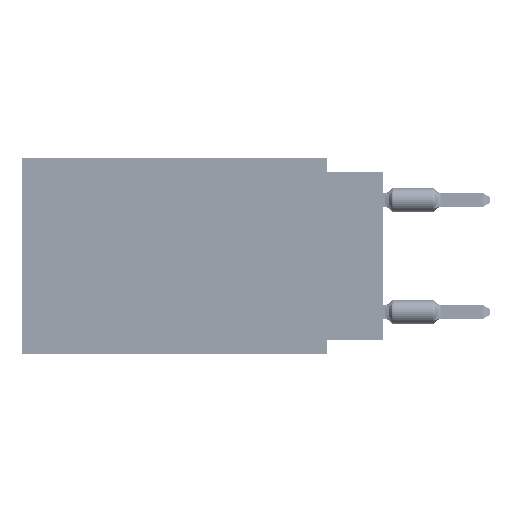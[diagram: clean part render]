
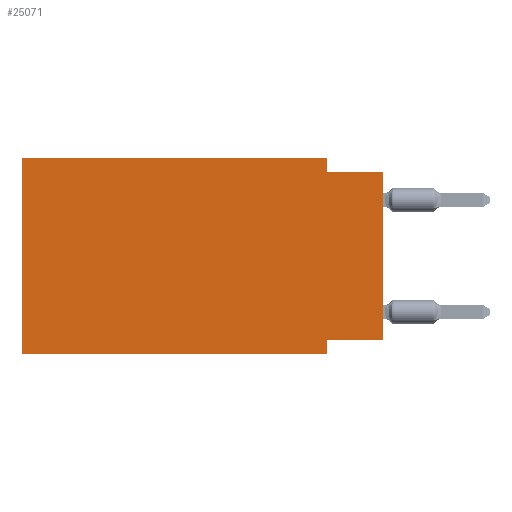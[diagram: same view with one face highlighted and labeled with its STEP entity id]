
A CAD part, left-side view. The second image highlights one B-rep face of the part: STEP entity #25071.
In plain terms, the highlighted planar face has unit normal (-1, 0, 0).
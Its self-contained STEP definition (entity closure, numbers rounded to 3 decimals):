
#673 = CARTESIAN_POINT ( 'NONE',  ( 0., 16.383, -8.89 ) ) ;
#1722 = EDGE_CURVE ( 'NONE', #19170, #26850, #45994, .T. ) ;
#2301 = EDGE_CURVE ( 'NONE', #38487, #80072, #85612, .T. ) ;
#2666 = LINE ( 'NONE', #11563, #86564 ) ;
#3224 = EDGE_CURVE ( 'NONE', #51161, #48623, #49148, .T. ) ;
#7296 = LINE ( 'NONE', #36738, #79432 ) ;
#8355 = DIRECTION ( 'NONE',  ( 0., -1., 0. ) ) ;
#9740 = EDGE_CURVE ( 'NONE', #73928, #40992, #46923, .T. ) ;
#11563 = CARTESIAN_POINT ( 'NONE',  ( 0., 16.383, 0. ) ) ;
#12191 = CARTESIAN_POINT ( 'NONE',  ( 0., 2.54, -8.255 ) ) ;
#13010 = EDGE_CURVE ( 'NONE', #80072, #48623, #7296, .T. ) ;
#15290 = FACE_OUTER_BOUND ( 'NONE', #47581, .T. ) ;
#19170 = VERTEX_POINT ( 'NONE', #38067 ) ;
#19643 = EDGE_CURVE ( 'NONE', #38487, #26850, #84244, .T. ) ;
#20157 = CARTESIAN_POINT ( 'NONE',  ( 0., 0., -0.635 ) ) ;
#23445 = VECTOR ( 'NONE', #8355, 1000. ) ;
#24925 = ORIENTED_EDGE ( 'NONE', *, *, #2301, .F. ) ;
#25053 = CARTESIAN_POINT ( 'NONE',  ( 0., 2.54, -8.89 ) ) ;
#25071 = ADVANCED_FACE ( 'NONE', ( #15290 ), #63773, .F. ) ;
#26850 = VERTEX_POINT ( 'NONE', #20157 ) ;
#27128 = CARTESIAN_POINT ( 'NONE',  ( 0., 2.54, 0. ) ) ;
#28039 = CARTESIAN_POINT ( 'NONE',  ( 0., 0., -8.255 ) ) ;
#30265 = DIRECTION ( 'NONE',  ( 0., 0., 1. ) ) ;
#31222 = VECTOR ( 'NONE', #57771, 1000. ) ;
#35587 = CARTESIAN_POINT ( 'NONE',  ( 0., 16.383, 0. ) ) ;
#36738 = CARTESIAN_POINT ( 'NONE',  ( 0., 2.54, -8.89 ) ) ;
#37115 = DIRECTION ( 'NONE',  ( 0., 0., 1. ) ) ;
#38067 = CARTESIAN_POINT ( 'NONE',  ( 0., 2.54, -0.635 ) ) ;
#38487 = VERTEX_POINT ( 'NONE', #28039 ) ;
#39197 = CARTESIAN_POINT ( 'NONE',  ( 0., 0., -0.635 ) ) ;
#40992 = VERTEX_POINT ( 'NONE', #27128 ) ;
#44279 = DIRECTION ( 'NONE',  ( 0., 0., -1. ) ) ;
#45994 = LINE ( 'NONE', #39197, #72410 ) ;
#46923 = LINE ( 'NONE', #52808, #84940 ) ;
#47581 = EDGE_LOOP ( 'NONE', ( #84273, #74457, #87370, #72584, #69758, #73638, #73192, #24925 ) ) ;
#48623 = VERTEX_POINT ( 'NONE', #25053 ) ;
#49148 = LINE ( 'NONE', #70440, #23445 ) ;
#49540 = EDGE_CURVE ( 'NONE', #51161, #73928, #2666, .T. ) ;
#50245 = DIRECTION ( 'NONE',  ( 0., 1., 0. ) ) ;
#51161 = VERTEX_POINT ( 'NONE', #673 ) ;
#51870 = CARTESIAN_POINT ( 'NONE',  ( 0., 2.54, 0. ) ) ;
#52808 = CARTESIAN_POINT ( 'NONE',  ( 0., 16.383, 0. ) ) ;
#57415 = CARTESIAN_POINT ( 'NONE',  ( 0., 16.383, 0. ) ) ;
#57771 = DIRECTION ( 'NONE',  ( 0., 0., -1. ) ) ;
#58594 = EDGE_CURVE ( 'NONE', #40992, #19170, #59118, .T. ) ;
#59118 = LINE ( 'NONE', #51870, #31222 ) ;
#63773 = PLANE ( 'NONE',  #71945 ) ;
#64251 = VECTOR ( 'NONE', #30265, 1000. ) ;
#64371 = DIRECTION ( 'NONE',  ( 0., 0., -1. ) ) ;
#64743 = CARTESIAN_POINT ( 'NONE',  ( 0., 0., -8.255 ) ) ;
#66845 = DIRECTION ( 'NONE',  ( 0., -1., 0. ) ) ;
#69758 = ORIENTED_EDGE ( 'NONE', *, *, #49540, .F. ) ;
#70440 = CARTESIAN_POINT ( 'NONE',  ( 0., 16.383, -8.89 ) ) ;
#71044 = CARTESIAN_POINT ( 'NONE',  ( 0., 0., 0. ) ) ;
#71945 = AXIS2_PLACEMENT_3D ( 'NONE', #57415, #85090, #44279 ) ;
#72410 = VECTOR ( 'NONE', #66845, 1000. ) ;
#72584 = ORIENTED_EDGE ( 'NONE', *, *, #9740, .F. ) ;
#73192 = ORIENTED_EDGE ( 'NONE', *, *, #13010, .F. ) ;
#73638 = ORIENTED_EDGE ( 'NONE', *, *, #3224, .T. ) ;
#73928 = VERTEX_POINT ( 'NONE', #35587 ) ;
#74457 = ORIENTED_EDGE ( 'NONE', *, *, #1722, .F. ) ;
#79432 = VECTOR ( 'NONE', #64371, 1000. ) ;
#80072 = VERTEX_POINT ( 'NONE', #12191 ) ;
#80495 = DIRECTION ( 'NONE',  ( 0., -1., 0. ) ) ;
#84244 = LINE ( 'NONE', #71044, #64251 ) ;
#84273 = ORIENTED_EDGE ( 'NONE', *, *, #19643, .T. ) ;
#84940 = VECTOR ( 'NONE', #80495, 1000. ) ;
#85090 = DIRECTION ( 'NONE',  ( 1., 0., 0. ) ) ;
#85564 = VECTOR ( 'NONE', #50245, 1000. ) ;
#85612 = LINE ( 'NONE', #64743, #85564 ) ;
#86564 = VECTOR ( 'NONE', #37115, 1000. ) ;
#87370 = ORIENTED_EDGE ( 'NONE', *, *, #58594, .F. ) ;
